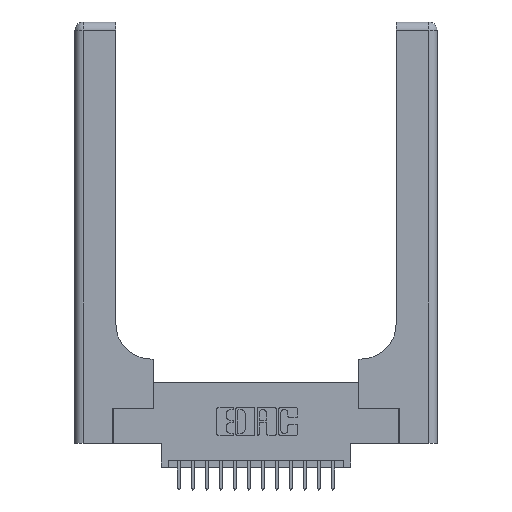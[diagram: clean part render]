
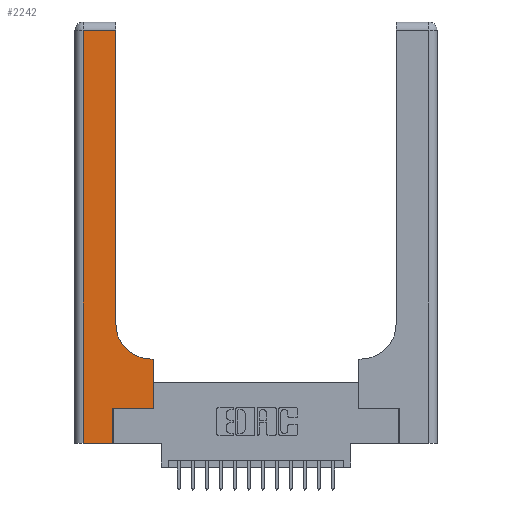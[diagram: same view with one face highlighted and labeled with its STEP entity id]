
A CAD part, top view. The second image highlights one B-rep face of the part: STEP entity #2242.
In plain terms, the highlighted planar face has unit normal (0, 0, 1).
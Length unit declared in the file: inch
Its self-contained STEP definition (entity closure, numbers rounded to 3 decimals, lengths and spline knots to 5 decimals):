
#397 = CARTESIAN_POINT ( 'NONE',  ( 0.2915, 3., 0.37 ) ) ;
#860 = CARTESIAN_POINT ( 'NONE',  ( 0., 0., 0.37 ) ) ;
#1106 = ORIENTED_EDGE ( 'NONE', *, *, #12860, .T. ) ;
#1851 = VECTOR ( 'NONE', #18390, 39.37008 ) ;
#2075 = CARTESIAN_POINT ( 'NONE',  ( 0.5585, 0.25, 0.37 ) ) ;
#2186 = ORIENTED_EDGE ( 'NONE', *, *, #12627, .T. ) ;
#2242 = ADVANCED_FACE ( 'NONE', ( #2974 ), #14129, .F. ) ;
#2331 = EDGE_CURVE ( 'NONE', #10810, #7958, #4268, .T. ) ;
#2568 = CARTESIAN_POINT ( 'NONE',  ( 0.269, 0., 0.37 ) ) ;
#2816 = CARTESIAN_POINT ( 'NONE',  ( 0.269, 0., 0.37 ) ) ;
#2871 = DIRECTION ( 'NONE',  ( -1., 0., 0. ) ) ;
#2974 = FACE_OUTER_BOUND ( 'NONE', #5191, .T. ) ;
#3234 = LINE ( 'NONE', #860, #1851 ) ;
#3639 = VERTEX_POINT ( 'NONE', #13850 ) ;
#3873 = EDGE_CURVE ( 'NONE', #10329, #5612, #8897, .T. ) ;
#3984 = DIRECTION ( 'NONE',  ( 0., 1., 0. ) ) ;
#4101 = VERTEX_POINT ( 'NONE', #16870 ) ;
#4107 = CARTESIAN_POINT ( 'NONE',  ( 0.06, 3., 0.37 ) ) ;
#4111 = VECTOR ( 'NONE', #18729, 39.37008 ) ;
#4268 = CIRCLE ( 'NONE', #16216, 0.25 ) ;
#4457 = VECTOR ( 'NONE', #13487, 39.37008 ) ;
#4775 = VERTEX_POINT ( 'NONE', #2816 ) ;
#4828 = EDGE_CURVE ( 'NONE', #13579, #3639, #8412, .T. ) ;
#4990 = CARTESIAN_POINT ( 'NONE',  ( 0.5415, 0.6, 0.37 ) ) ;
#5191 = EDGE_LOOP ( 'NONE', ( #16397, #7434, #16578, #9038, #2186, #1106, #11214, #15569, #13404 ) ) ;
#5612 = VERTEX_POINT ( 'NONE', #9126 ) ;
#5993 = CARTESIAN_POINT ( 'NONE',  ( 0.2915, 0.85, 0.37 ) ) ;
#6012 = VECTOR ( 'NONE', #6604, 39.37008 ) ;
#6039 = VECTOR ( 'NONE', #2871, 39.37008 ) ;
#6604 = DIRECTION ( 'NONE',  ( -1., 0., 0. ) ) ;
#6824 = DIRECTION ( 'NONE',  ( 0., 0., -1. ) ) ;
#6854 = CARTESIAN_POINT ( 'NONE',  ( 0.2915, 0.6, 0.37 ) ) ;
#7060 = DIRECTION ( 'NONE',  ( 1., 0., 0. ) ) ;
#7357 = DIRECTION ( 'NONE',  ( 0., 1., 0. ) ) ;
#7434 = ORIENTED_EDGE ( 'NONE', *, *, #16110, .T. ) ;
#7958 = VERTEX_POINT ( 'NONE', #5993 ) ;
#8412 = LINE ( 'NONE', #8771, #11844 ) ;
#8433 = VECTOR ( 'NONE', #15059, 39.37008 ) ;
#8641 = DIRECTION ( 'NONE',  ( 0., 0., -1. ) ) ;
#8771 = CARTESIAN_POINT ( 'NONE',  ( 0.5585, 0.25, 0.37 ) ) ;
#8897 = LINE ( 'NONE', #4107, #4111 ) ;
#9038 = ORIENTED_EDGE ( 'NONE', *, *, #18646, .T. ) ;
#9126 = CARTESIAN_POINT ( 'NONE',  ( 0.06, 0., 0.37 ) ) ;
#9267 = VECTOR ( 'NONE', #3984, 39.37008 ) ;
#9497 = AXIS2_PLACEMENT_3D ( 'NONE', #18512, #6824, #17049 ) ;
#9916 = LINE ( 'NONE', #6854, #6012 ) ;
#9991 = VERTEX_POINT ( 'NONE', #18699 ) ;
#10329 = VERTEX_POINT ( 'NONE', #18794 ) ;
#10517 = EDGE_CURVE ( 'NONE', #7958, #4101, #14643, .T. ) ;
#10810 = VERTEX_POINT ( 'NONE', #4990 ) ;
#10860 = LINE ( 'NONE', #15931, #6039 ) ;
#11214 = ORIENTED_EDGE ( 'NONE', *, *, #4828, .T. ) ;
#11844 = VECTOR ( 'NONE', #7357, 39.37008 ) ;
#12627 = EDGE_CURVE ( 'NONE', #4775, #9991, #13157, .T. ) ;
#12860 = EDGE_CURVE ( 'NONE', #9991, #13579, #18403, .T. ) ;
#13157 = LINE ( 'NONE', #2568, #9267 ) ;
#13404 = ORIENTED_EDGE ( 'NONE', *, *, #2331, .T. ) ;
#13487 = DIRECTION ( 'NONE',  ( 1., 0., 0. ) ) ;
#13579 = VERTEX_POINT ( 'NONE', #2075 ) ;
#13850 = CARTESIAN_POINT ( 'NONE',  ( 0.5585, 0.6, 0.37 ) ) ;
#14116 = EDGE_CURVE ( 'NONE', #3639, #10810, #9916, .T. ) ;
#14129 = PLANE ( 'NONE',  #9497 ) ;
#14643 = LINE ( 'NONE', #397, #8433 ) ;
#15059 = DIRECTION ( 'NONE',  ( 0., 1., 0. ) ) ;
#15569 = ORIENTED_EDGE ( 'NONE', *, *, #14116, .T. ) ;
#15931 = CARTESIAN_POINT ( 'NONE',  ( 0., 2.94, 0.37 ) ) ;
#16110 = EDGE_CURVE ( 'NONE', #4101, #10329, #10860, .T. ) ;
#16216 = AXIS2_PLACEMENT_3D ( 'NONE', #17405, #8641, #7060 ) ;
#16351 = CARTESIAN_POINT ( 'NONE',  ( 0.269, 0.25, 0.37 ) ) ;
#16397 = ORIENTED_EDGE ( 'NONE', *, *, #10517, .T. ) ;
#16578 = ORIENTED_EDGE ( 'NONE', *, *, #3873, .T. ) ;
#16870 = CARTESIAN_POINT ( 'NONE',  ( 0.2915, 2.94, 0.37 ) ) ;
#17049 = DIRECTION ( 'NONE',  ( -1., 0., 0. ) ) ;
#17405 = CARTESIAN_POINT ( 'NONE',  ( 0.5415, 0.85, 0.37 ) ) ;
#18390 = DIRECTION ( 'NONE',  ( 1., 0., 0. ) ) ;
#18403 = LINE ( 'NONE', #16351, #4457 ) ;
#18512 = CARTESIAN_POINT ( 'NONE',  ( 0., 3., 0.37 ) ) ;
#18646 = EDGE_CURVE ( 'NONE', #5612, #4775, #3234, .T. ) ;
#18699 = CARTESIAN_POINT ( 'NONE',  ( 0.269, 0.25, 0.37 ) ) ;
#18729 = DIRECTION ( 'NONE',  ( 0., -1., 0. ) ) ;
#18794 = CARTESIAN_POINT ( 'NONE',  ( 0.06, 2.94, 0.37 ) ) ;
